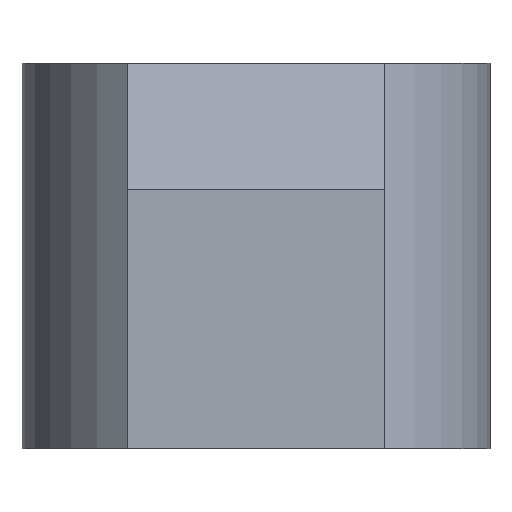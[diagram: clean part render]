
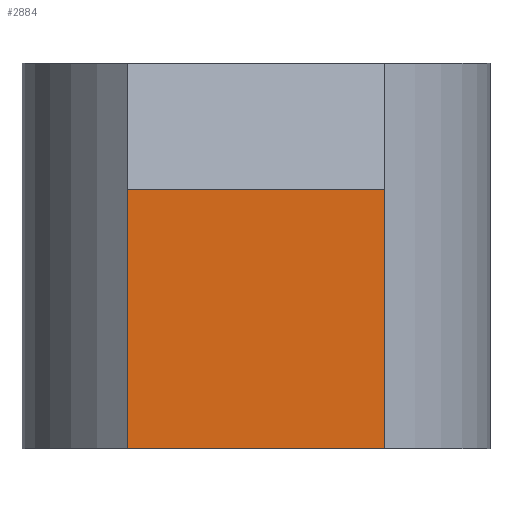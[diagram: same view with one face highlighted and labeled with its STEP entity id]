
A CAD part, front view. The second image highlights one B-rep face of the part: STEP entity #2884.
In plain terms, the highlighted planar face has unit normal (0, -1, 0).
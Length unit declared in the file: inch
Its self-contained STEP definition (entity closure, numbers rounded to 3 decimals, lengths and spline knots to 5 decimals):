
#51 = VERTEX_POINT ( 'NONE', #2672 ) ;
#252 = VECTOR ( 'NONE', #3874, 39.37008 ) ;
#308 = CARTESIAN_POINT ( 'NONE',  ( -1.1175, 0.065, 0. ) ) ;
#327 = DIRECTION ( 'NONE',  ( 0., 1., 0. ) ) ;
#363 = ORIENTED_EDGE ( 'NONE', *, *, #3576, .T. ) ;
#608 = AXIS2_PLACEMENT_3D ( 'NONE', #3004, #327, #1046 ) ;
#723 = DIRECTION ( 'NONE',  ( 0., 0., -1. ) ) ;
#777 = VERTEX_POINT ( 'NONE', #308 ) ;
#1046 = DIRECTION ( 'NONE',  ( -1., 0., 0. ) ) ;
#1056 = CARTESIAN_POINT ( 'NONE',  ( -1.3675, 0.065, 0.25246 ) ) ;
#1116 = EDGE_CURVE ( 'NONE', #2448, #3077, #1379, .T. ) ;
#1247 = FACE_OUTER_BOUND ( 'NONE', #3996, .T. ) ;
#1379 = LINE ( 'NONE', #1565, #1586 ) ;
#1565 = CARTESIAN_POINT ( 'NONE',  ( -1.1175, 0.065, 0.25246 ) ) ;
#1586 = VECTOR ( 'NONE', #3844, 39.37008 ) ;
#1792 = ORIENTED_EDGE ( 'NONE', *, *, #2235, .T. ) ;
#1818 = CARTESIAN_POINT ( 'NONE',  ( -1.1175, 0.065, 0.25246 ) ) ;
#2189 = ORIENTED_EDGE ( 'NONE', *, *, #1116, .T. ) ;
#2235 = EDGE_CURVE ( 'NONE', #51, #777, #2869, .T. ) ;
#2330 = CARTESIAN_POINT ( 'NONE',  ( -1.3675, 0.065, 0.375 ) ) ;
#2420 = VECTOR ( 'NONE', #723, 39.37008 ) ;
#2448 = VERTEX_POINT ( 'NONE', #1818 ) ;
#2591 = CARTESIAN_POINT ( 'NONE',  ( -1.1175, 0.065, 0. ) ) ;
#2672 = CARTESIAN_POINT ( 'NONE',  ( -1.3675, 0.065, 0. ) ) ;
#2734 = VECTOR ( 'NONE', #3629, 39.37008 ) ;
#2869 = LINE ( 'NONE', #2591, #252 ) ;
#2884 = ADVANCED_FACE ( 'NONE', ( #1247 ), #2975, .F. ) ;
#2975 = PLANE ( 'NONE',  #608 ) ;
#3004 = CARTESIAN_POINT ( 'NONE',  ( -1.1175, 0.065, 0.375 ) ) ;
#3077 = VERTEX_POINT ( 'NONE', #1056 ) ;
#3341 = EDGE_CURVE ( 'NONE', #2448, #777, #3497, .T. ) ;
#3359 = CARTESIAN_POINT ( 'NONE',  ( -1.1175, 0.065, 0.375 ) ) ;
#3447 = LINE ( 'NONE', #2330, #2734 ) ;
#3497 = LINE ( 'NONE', #3359, #2420 ) ;
#3576 = EDGE_CURVE ( 'NONE', #3077, #51, #3447, .T. ) ;
#3629 = DIRECTION ( 'NONE',  ( 0., 0., -1. ) ) ;
#3844 = DIRECTION ( 'NONE',  ( -1., 0., 0. ) ) ;
#3874 = DIRECTION ( 'NONE',  ( 1., 0., 0. ) ) ;
#3996 = EDGE_LOOP ( 'NONE', ( #4044, #2189, #363, #1792 ) ) ;
#4044 = ORIENTED_EDGE ( 'NONE', *, *, #3341, .F. ) ;
